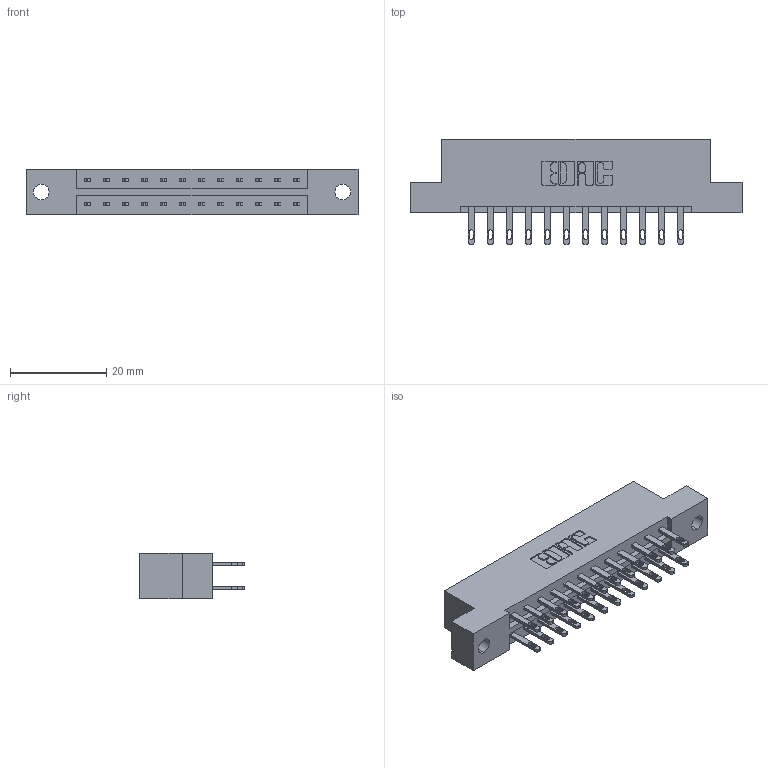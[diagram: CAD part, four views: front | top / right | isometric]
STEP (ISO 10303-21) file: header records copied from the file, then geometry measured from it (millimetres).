
FILE_DESCRIPTION (( 'STEP AP203' ), '1' );
FILE_NAME ('833-024-500-202.STEP', '2020-06-01T19:56:48', ( '' ), ( '' ), 'SwSTEP 2.0', 'SolidWorks 2020', '' );
FILE_SCHEMA (( 'CONFIG_CONTROL_DESIGN' ));
Length unit declared in the file: inch
Products named in the file (3): 833 Part_Flush - .128 Dia; 345-292-001_345-293-100; 833-024-500-202
Assembly tree (25 placements, depth 2):
  833-024-500-202
    833 Part_Flush - .128 Dia
    345-292-001_345-293-100  x24
Bounding box: 69.09 x 21.85 x 9.4 mm (x, y, z)
Volume: 6809.6 mm3; surface area: 7719 mm2
Topology: 25 solids, 25 shells, 1266 faces, 3839 edges, 2558 vertices
Faces by surface type: plane 790, cylinder 476
Entity records: 11533 total; most frequent: CARTESIAN_POINT 1946, ORIENTED_EDGE 1882, DIRECTION 1717, EDGE_CURVE 941, LINE 809, VECTOR 809, VERTEX_POINT 626, AXIS2_PLACEMENT_3D 454
